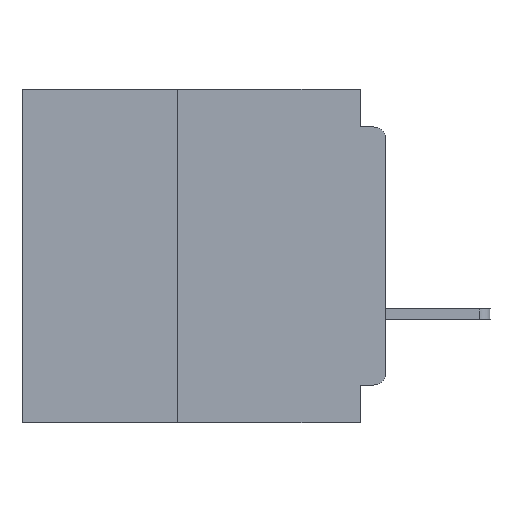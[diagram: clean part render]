
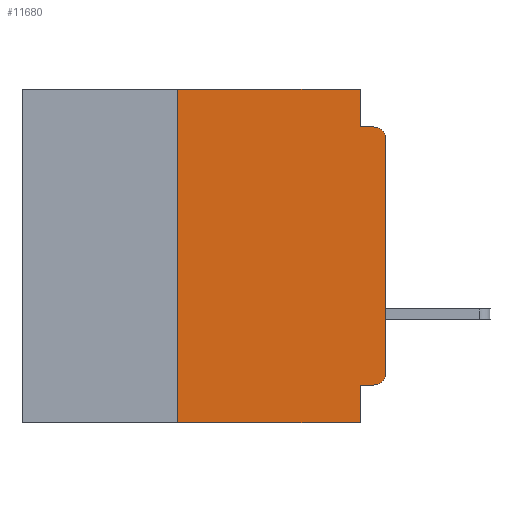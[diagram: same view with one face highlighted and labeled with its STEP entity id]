
A CAD part, left-side view. The second image highlights one B-rep face of the part: STEP entity #11680.
In plain terms, the highlighted planar face has unit normal (-1, 0, 0).
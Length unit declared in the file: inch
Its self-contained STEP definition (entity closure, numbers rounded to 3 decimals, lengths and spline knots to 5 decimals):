
#476 = VECTOR ( 'NONE', #36541, 39.37008 ) ;
#936 = EDGE_CURVE ( 'NONE', #6571, #52681, #24197, .T. ) ;
#1214 = DIRECTION ( 'NONE',  ( 0., 0., -1. ) ) ;
#1638 = DIRECTION ( 'NONE',  ( 0., 0., -1. ) ) ;
#2685 = DIRECTION ( 'NONE',  ( 0., 0., 1. ) ) ;
#2797 = CIRCLE ( 'NONE', #24682, 0.015 ) ;
#3643 = VERTEX_POINT ( 'NONE', #53632 ) ;
#3959 = VERTEX_POINT ( 'NONE', #6536 ) ;
#4776 = VERTEX_POINT ( 'NONE', #30461 ) ;
#5616 = ORIENTED_EDGE ( 'NONE', *, *, #8508, .T. ) ;
#5705 = DIRECTION ( 'NONE',  ( 1., 0., 0. ) ) ;
#6175 = DIRECTION ( 'NONE',  ( 0., 0., -1. ) ) ;
#6356 = CARTESIAN_POINT ( 'NONE',  ( 0., 0., -0.355 ) ) ;
#6536 = CARTESIAN_POINT ( 'NONE',  ( 0., 0.015, -0.355 ) ) ;
#6571 = VERTEX_POINT ( 'NONE', #14378 ) ;
#6647 = EDGE_LOOP ( 'NONE', ( #49377, #38707, #58251, #55520, #22377, #34313, #56782, #16874, #33401, #5616 ) ) ;
#8508 = EDGE_CURVE ( 'NONE', #3959, #16213, #2797, .T. ) ;
#8820 = CARTESIAN_POINT ( 'NONE',  ( 0., 0.015, -0.045 ) ) ;
#9583 = CARTESIAN_POINT ( 'NONE',  ( 0., 0.031, -0.4 ) ) ;
#10015 = LINE ( 'NONE', #29716, #21977 ) ;
#10061 = CARTESIAN_POINT ( 'NONE',  ( 0., 0.437, 0. ) ) ;
#10220 = EDGE_CURVE ( 'NONE', #14223, #52681, #12593, .T. ) ;
#10316 = CARTESIAN_POINT ( 'NONE',  ( 0., 0.031, -0.355 ) ) ;
#10608 = EDGE_CURVE ( 'NONE', #23676, #33629, #15357, .T. ) ;
#11270 = LINE ( 'NONE', #6356, #45700 ) ;
#11680 = ADVANCED_FACE ( 'NONE', ( #26487 ), #23637, .F. ) ;
#12593 = LINE ( 'NONE', #50026, #476 ) ;
#12914 = EDGE_CURVE ( 'NONE', #4776, #14223, #51504, .T. ) ;
#14111 = EDGE_CURVE ( 'NONE', #15514, #33629, #35136, .T. ) ;
#14223 = VERTEX_POINT ( 'NONE', #27150 ) ;
#14378 = CARTESIAN_POINT ( 'NONE',  ( 0., 0., -0.06 ) ) ;
#14985 = VECTOR ( 'NONE', #56157, 39.37008 ) ;
#15357 = LINE ( 'NONE', #21400, #25914 ) ;
#15514 = VERTEX_POINT ( 'NONE', #10316 ) ;
#16213 = VERTEX_POINT ( 'NONE', #55705 ) ;
#16874 = ORIENTED_EDGE ( 'NONE', *, *, #14111, .F. ) ;
#17384 = CARTESIAN_POINT ( 'NONE',  ( 0., 0.25, -0.4 ) ) ;
#20303 = DIRECTION ( 'NONE',  ( 0., 0., 1. ) ) ;
#21400 = CARTESIAN_POINT ( 'NONE',  ( 0., 0.437, -0.4 ) ) ;
#21977 = VECTOR ( 'NONE', #2685, 39.37008 ) ;
#22034 = EDGE_CURVE ( 'NONE', #16213, #6571, #24981, .T. ) ;
#22377 = ORIENTED_EDGE ( 'NONE', *, *, #55408, .F. ) ;
#23637 = PLANE ( 'NONE',  #52531 ) ;
#23676 = VERTEX_POINT ( 'NONE', #17384 ) ;
#23758 = CARTESIAN_POINT ( 'NONE',  ( 0., 0.031, -0.4 ) ) ;
#24197 = CIRCLE ( 'NONE', #25020, 0.015 ) ;
#24646 = CARTESIAN_POINT ( 'NONE',  ( 0., 0., 0. ) ) ;
#24682 = AXIS2_PLACEMENT_3D ( 'NONE', #55482, #28699, #1638 ) ;
#24981 = LINE ( 'NONE', #24646, #50184 ) ;
#25020 = AXIS2_PLACEMENT_3D ( 'NONE', #28711, #28632, #28044 ) ;
#25312 = EDGE_CURVE ( 'NONE', #3959, #15514, #11270, .T. ) ;
#25914 = VECTOR ( 'NONE', #48425, 39.37008 ) ;
#26487 = FACE_OUTER_BOUND ( 'NONE', #6647, .T. ) ;
#27150 = CARTESIAN_POINT ( 'NONE',  ( 0., 0.031, -0.045 ) ) ;
#28044 = DIRECTION ( 'NONE',  ( 0., 0., -1. ) ) ;
#28632 = DIRECTION ( 'NONE',  ( -1., 0., 0. ) ) ;
#28699 = DIRECTION ( 'NONE',  ( -1., 0., 0. ) ) ;
#28711 = CARTESIAN_POINT ( 'NONE',  ( 0., 0.015, -0.06 ) ) ;
#29716 = CARTESIAN_POINT ( 'NONE',  ( 0., 0.25, -0.4 ) ) ;
#30461 = CARTESIAN_POINT ( 'NONE',  ( 0., 0.031, 0. ) ) ;
#33110 = CARTESIAN_POINT ( 'NONE',  ( 0., 0.031, 0. ) ) ;
#33301 = DIRECTION ( 'NONE',  ( 0., 1., 0. ) ) ;
#33401 = ORIENTED_EDGE ( 'NONE', *, *, #25312, .F. ) ;
#33629 = VERTEX_POINT ( 'NONE', #9583 ) ;
#34313 = ORIENTED_EDGE ( 'NONE', *, *, #35293, .F. ) ;
#35136 = LINE ( 'NONE', #23758, #45666 ) ;
#35293 = EDGE_CURVE ( 'NONE', #23676, #3643, #10015, .T. ) ;
#36541 = DIRECTION ( 'NONE',  ( 0., -1., 0. ) ) ;
#37144 = DIRECTION ( 'NONE',  ( 0., 0., -1. ) ) ;
#38707 = ORIENTED_EDGE ( 'NONE', *, *, #936, .T. ) ;
#38879 = LINE ( 'NONE', #51646, #14985 ) ;
#39650 = VECTOR ( 'NONE', #6175, 39.37008 ) ;
#45666 = VECTOR ( 'NONE', #1214, 39.37008 ) ;
#45700 = VECTOR ( 'NONE', #33301, 39.37008 ) ;
#48425 = DIRECTION ( 'NONE',  ( 0., -1., 0. ) ) ;
#49377 = ORIENTED_EDGE ( 'NONE', *, *, #22034, .T. ) ;
#50026 = CARTESIAN_POINT ( 'NONE',  ( 0., 0., -0.045 ) ) ;
#50184 = VECTOR ( 'NONE', #20303, 39.37008 ) ;
#51504 = LINE ( 'NONE', #33110, #39650 ) ;
#51646 = CARTESIAN_POINT ( 'NONE',  ( 0., 0.437, 0. ) ) ;
#52531 = AXIS2_PLACEMENT_3D ( 'NONE', #10061, #5705, #37144 ) ;
#52681 = VERTEX_POINT ( 'NONE', #8820 ) ;
#53632 = CARTESIAN_POINT ( 'NONE',  ( 0., 0.25, 0. ) ) ;
#55408 = EDGE_CURVE ( 'NONE', #3643, #4776, #38879, .T. ) ;
#55482 = CARTESIAN_POINT ( 'NONE',  ( 0., 0.015, -0.34 ) ) ;
#55520 = ORIENTED_EDGE ( 'NONE', *, *, #12914, .F. ) ;
#55705 = CARTESIAN_POINT ( 'NONE',  ( 0., 0., -0.34 ) ) ;
#56157 = DIRECTION ( 'NONE',  ( 0., -1., 0. ) ) ;
#56782 = ORIENTED_EDGE ( 'NONE', *, *, #10608, .T. ) ;
#58251 = ORIENTED_EDGE ( 'NONE', *, *, #10220, .F. ) ;
